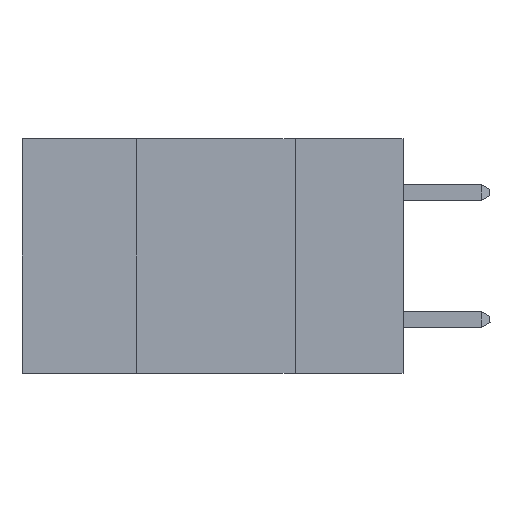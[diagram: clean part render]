
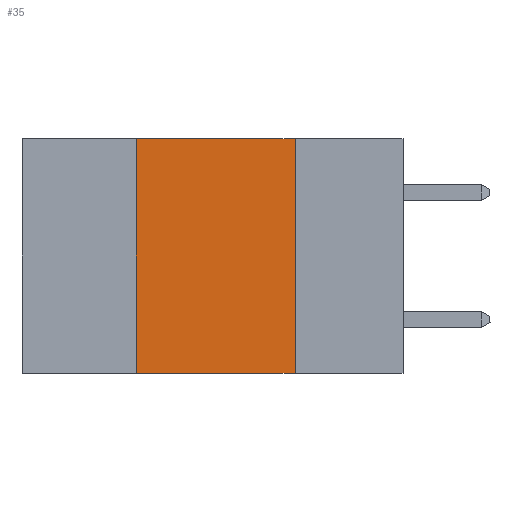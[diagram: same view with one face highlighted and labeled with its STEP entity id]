
A CAD part, left-side view. The second image highlights one B-rep face of the part: STEP entity #35.
In plain terms, the highlighted planar face has unit normal (-1, 0, 0).
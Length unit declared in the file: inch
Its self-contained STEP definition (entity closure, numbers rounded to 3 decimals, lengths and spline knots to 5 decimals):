
#35 = ADVANCED_FACE ( 'NONE', ( #12039 ), #10812, .F. ) ;
#687 = VECTOR ( 'NONE', #17043, 39.37008 ) ;
#1989 = VERTEX_POINT ( 'NONE', #9904 ) ;
#1997 = DIRECTION ( 'NONE',  ( 0., 0., -1. ) ) ;
#2130 = ORIENTED_EDGE ( 'NONE', *, *, #14531, .F. ) ;
#2586 = AXIS2_PLACEMENT_3D ( 'NONE', #5623, #4529, #11377 ) ;
#3453 = CARTESIAN_POINT ( 'NONE',  ( 0., 0.17, 0. ) ) ;
#4529 = DIRECTION ( 'NONE',  ( 1., 0., 0. ) ) ;
#4728 = VECTOR ( 'NONE', #1997, 39.37008 ) ;
#4787 = VECTOR ( 'NONE', #9058, 39.37008 ) ;
#5623 = CARTESIAN_POINT ( 'NONE',  ( 0., 0.6, 0. ) ) ;
#5882 = ORIENTED_EDGE ( 'NONE', *, *, #17211, .T. ) ;
#7816 = CARTESIAN_POINT ( 'NONE',  ( 0., 0.17, -0.37 ) ) ;
#8142 = EDGE_CURVE ( 'NONE', #13394, #15044, #8213, .T. ) ;
#8213 = LINE ( 'NONE', #3453, #4728 ) ;
#8508 = LINE ( 'NONE', #15717, #687 ) ;
#8744 = VERTEX_POINT ( 'NONE', #11262 ) ;
#9058 = DIRECTION ( 'NONE',  ( 0., 0., 1. ) ) ;
#9904 = CARTESIAN_POINT ( 'NONE',  ( 0., 0.42, 0. ) ) ;
#10257 = CARTESIAN_POINT ( 'NONE',  ( 0., 0.6, 0. ) ) ;
#10495 = VECTOR ( 'NONE', #11531, 39.37008 ) ;
#10812 = PLANE ( 'NONE',  #2586 ) ;
#11262 = CARTESIAN_POINT ( 'NONE',  ( 0., 0.42, -0.37 ) ) ;
#11377 = DIRECTION ( 'NONE',  ( 0., 0., -1. ) ) ;
#11531 = DIRECTION ( 'NONE',  ( 0., -1., 0. ) ) ;
#11583 = EDGE_LOOP ( 'NONE', ( #12324, #15944, #2130, #5882 ) ) ;
#12039 = FACE_OUTER_BOUND ( 'NONE', #11583, .T. ) ;
#12324 = ORIENTED_EDGE ( 'NONE', *, *, #8142, .F. ) ;
#13140 = LINE ( 'NONE', #10257, #10495 ) ;
#13394 = VERTEX_POINT ( 'NONE', #17226 ) ;
#13759 = EDGE_CURVE ( 'NONE', #1989, #13394, #13140, .T. ) ;
#14272 = CARTESIAN_POINT ( 'NONE',  ( 0., 0.42, 0. ) ) ;
#14531 = EDGE_CURVE ( 'NONE', #8744, #1989, #14830, .T. ) ;
#14830 = LINE ( 'NONE', #14272, #4787 ) ;
#15044 = VERTEX_POINT ( 'NONE', #7816 ) ;
#15717 = CARTESIAN_POINT ( 'NONE',  ( 0., 0.6, -0.37 ) ) ;
#15944 = ORIENTED_EDGE ( 'NONE', *, *, #13759, .F. ) ;
#17043 = DIRECTION ( 'NONE',  ( 0., -1., 0. ) ) ;
#17211 = EDGE_CURVE ( 'NONE', #8744, #15044, #8508, .T. ) ;
#17226 = CARTESIAN_POINT ( 'NONE',  ( 0., 0.17, 0. ) ) ;
